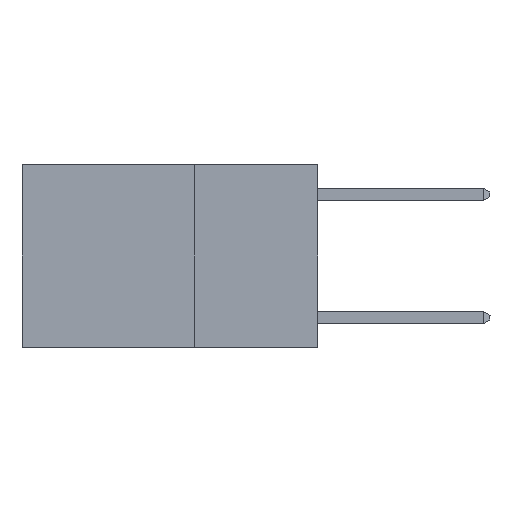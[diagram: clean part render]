
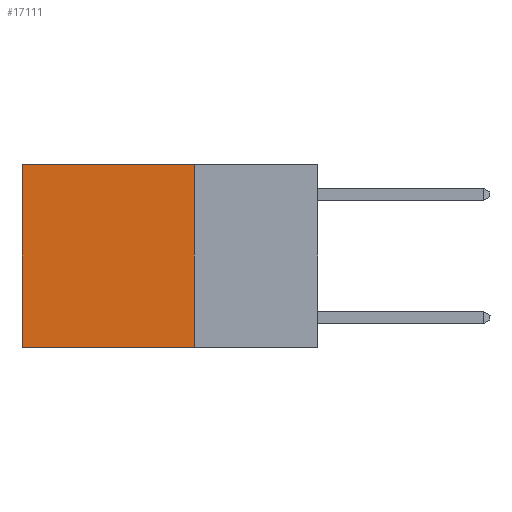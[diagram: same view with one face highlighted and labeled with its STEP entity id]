
A CAD part, left-side view. The second image highlights one B-rep face of the part: STEP entity #17111.
In plain terms, the highlighted planar face has unit normal (-1, 0, 0).
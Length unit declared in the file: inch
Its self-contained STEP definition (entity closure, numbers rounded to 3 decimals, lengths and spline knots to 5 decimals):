
#3565 = CARTESIAN_POINT ( 'NONE',  ( 0.2625, 0.25, 0. ) ) ;
#4130 = LINE ( 'NONE', #15582, #16755 ) ;
#5814 = CARTESIAN_POINT ( 'NONE',  ( 0.2625, 0.25, 0. ) ) ;
#6922 = VERTEX_POINT ( 'NONE', #12698 ) ;
#6985 = VECTOR ( 'NONE', #26014, 39.37008 ) ;
#7189 = DIRECTION ( 'NONE',  ( 0., 0., -1. ) ) ;
#8570 = PLANE ( 'NONE',  #13738 ) ;
#10136 = EDGE_CURVE ( 'NONE', #17623, #17840, #16367, .T. ) ;
#11578 = EDGE_LOOP ( 'NONE', ( #29018, #21064, #12711, #14516 ) ) ;
#12375 = CARTESIAN_POINT ( 'NONE',  ( 0.2625, 0.6, -0.37 ) ) ;
#12698 = CARTESIAN_POINT ( 'NONE',  ( 0.2625, 0.25, -0.37 ) ) ;
#12711 = ORIENTED_EDGE ( 'NONE', *, *, #21796, .F. ) ;
#13655 = DIRECTION ( 'NONE',  ( 0., 0., -1. ) ) ;
#13738 = AXIS2_PLACEMENT_3D ( 'NONE', #26075, #28473, #13655 ) ;
#14516 = ORIENTED_EDGE ( 'NONE', *, *, #10136, .T. ) ;
#14719 = CARTESIAN_POINT ( 'NONE',  ( 0.2625, 0.6, 0. ) ) ;
#14785 = FACE_OUTER_BOUND ( 'NONE', #11578, .T. ) ;
#15582 = CARTESIAN_POINT ( 'NONE',  ( 0.2625, 0.25, -0.37 ) ) ;
#15766 = VECTOR ( 'NONE', #7189, 39.37008 ) ;
#16367 = LINE ( 'NONE', #19470, #21464 ) ;
#16755 = VECTOR ( 'NONE', #27989, 39.37008 ) ;
#17111 = ADVANCED_FACE ( 'NONE', ( #14785 ), #8570, .F. ) ;
#17351 = LINE ( 'NONE', #14719, #15766 ) ;
#17623 = VERTEX_POINT ( 'NONE', #5814 ) ;
#17840 = VERTEX_POINT ( 'NONE', #19152 ) ;
#19152 = CARTESIAN_POINT ( 'NONE',  ( 0.2625, 0.6, 0. ) ) ;
#19360 = DIRECTION ( 'NONE',  ( 0., 1., 0. ) ) ;
#19470 = CARTESIAN_POINT ( 'NONE',  ( 0.2625, 0.25, 0. ) ) ;
#21064 = ORIENTED_EDGE ( 'NONE', *, *, #31666, .F. ) ;
#21464 = VECTOR ( 'NONE', #19360, 39.37008 ) ;
#21796 = EDGE_CURVE ( 'NONE', #17623, #6922, #27641, .T. ) ;
#26014 = DIRECTION ( 'NONE',  ( 0., 0., -1. ) ) ;
#26075 = CARTESIAN_POINT ( 'NONE',  ( 0.2625, 0.25, 0. ) ) ;
#27641 = LINE ( 'NONE', #3565, #6985 ) ;
#27989 = DIRECTION ( 'NONE',  ( 0., 1., 0. ) ) ;
#28144 = EDGE_CURVE ( 'NONE', #17840, #30134, #17351, .T. ) ;
#28473 = DIRECTION ( 'NONE',  ( 1., 0., 0. ) ) ;
#29018 = ORIENTED_EDGE ( 'NONE', *, *, #28144, .T. ) ;
#30134 = VERTEX_POINT ( 'NONE', #12375 ) ;
#31666 = EDGE_CURVE ( 'NONE', #6922, #30134, #4130, .T. ) ;
